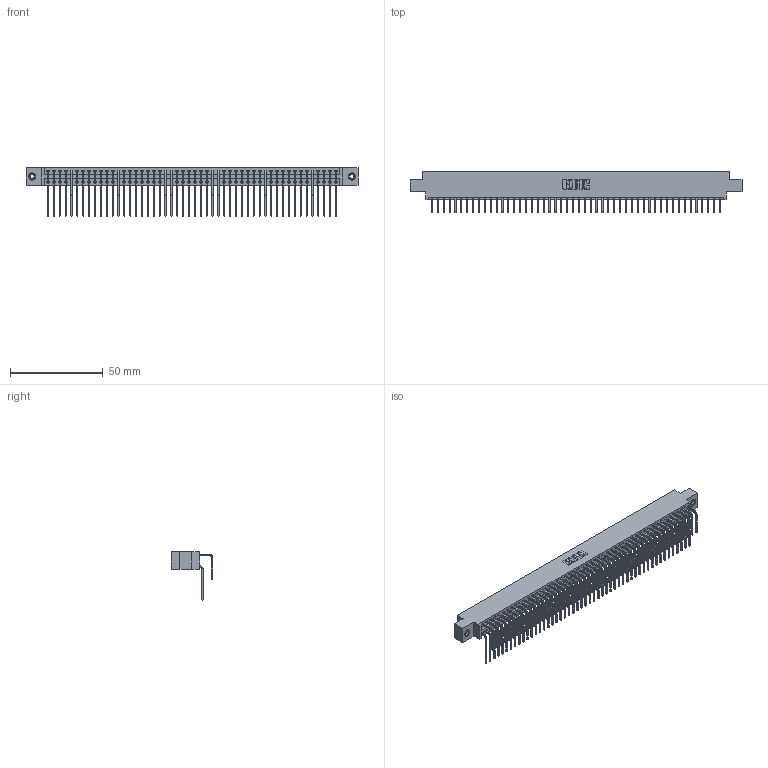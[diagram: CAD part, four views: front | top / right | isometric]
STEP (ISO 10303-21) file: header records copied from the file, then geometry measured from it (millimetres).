
FILE_DESCRIPTION (( 'STEP AP203' ), '1' );
FILE_NAME ('396-100-558-808.STEP', '2018-09-14T08:16:01', ( '' ), ( '' ), 'SwSTEP 2.0', 'SolidWorks 2016', '' );
FILE_SCHEMA (( 'CONFIG_CONTROL_DESIGN' ));
Length unit declared in the file: inch
Products named in the file (5): 345-292-001_558 559 Tail - 1; 345-292-001_558 Tail - 2; 345-250-001_345-250-003-102; 396-100-558-808; 346 Part_0.170 Offset - 0.156 Dia-TI
Assembly tree (103 placements, depth 2):
  396-100-558-808
    346 Part_0.170 Offset - 0.156 Dia-TI
    345-292-001_558 559 Tail - 1  x50
    345-292-001_558 Tail - 2  x50
    345-250-001_345-250-003-102  x2
Bounding box: 179.32 x 22.16 x 26.16 mm (x, y, z)
Volume: 17964.2 mm3; surface area: 27785.9 mm2
Topology: 103 solids, 103 shells, 5586 faces, 16577 edges, 10910 vertices
Faces by surface type: plane 3812, cylinder 1758, cone 12, torus 4
Entity records: 34656 total; most frequent: CARTESIAN_POINT 5738, ORIENTED_EDGE 5614, DIRECTION 5105, EDGE_CURVE 2807, LINE 2415, VECTOR 2415, VERTEX_POINT 1864, AXIS2_PLACEMENT_3D 1345
